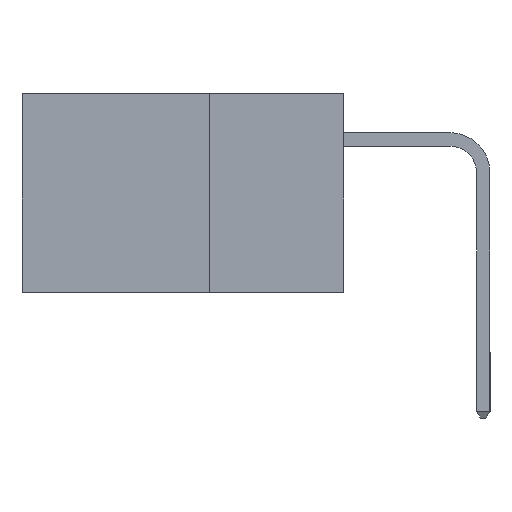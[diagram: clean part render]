
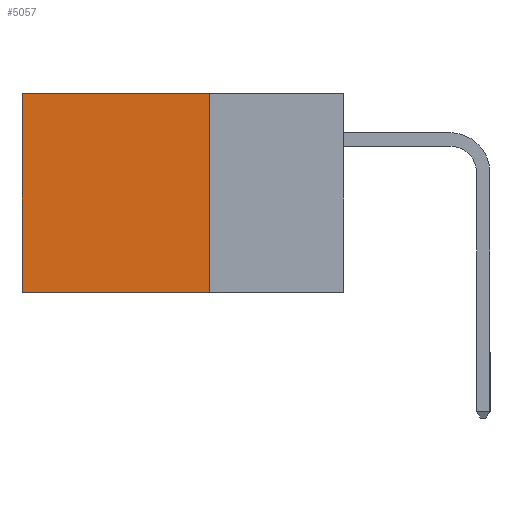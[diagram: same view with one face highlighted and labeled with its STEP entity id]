
A CAD part, left-side view. The second image highlights one B-rep face of the part: STEP entity #5057.
In plain terms, the highlighted planar face has unit normal (-1, 0, 0).
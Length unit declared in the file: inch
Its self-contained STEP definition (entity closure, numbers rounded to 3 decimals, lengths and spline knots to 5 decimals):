
#178 = CARTESIAN_POINT ( 'NONE',  ( 0.2615, 0.6, -0.37 ) ) ;
#509 = CARTESIAN_POINT ( 'NONE',  ( 0.2615, 0.6, 0. ) ) ;
#1676 = DIRECTION ( 'NONE',  ( 0., 0., -1. ) ) ;
#1909 = VERTEX_POINT ( 'NONE', #21114 ) ;
#2066 = LINE ( 'NONE', #12720, #18603 ) ;
#3176 = LINE ( 'NONE', #20677, #4703 ) ;
#3280 = CARTESIAN_POINT ( 'NONE',  ( 0.2615, 0.25, -0.37 ) ) ;
#4654 = DIRECTION ( 'NONE',  ( 0., 1., 0. ) ) ;
#4703 = VECTOR ( 'NONE', #17022, 39.37008 ) ;
#5057 = ADVANCED_FACE ( 'NONE', ( #5669 ), #10710, .F. ) ;
#5129 = EDGE_LOOP ( 'NONE', ( #5294, #18000, #10299, #13114 ) ) ;
#5294 = ORIENTED_EDGE ( 'NONE', *, *, #8417, .T. ) ;
#5669 = FACE_OUTER_BOUND ( 'NONE', #5129, .T. ) ;
#7840 = VECTOR ( 'NONE', #4654, 39.37008 ) ;
#8417 = EDGE_CURVE ( 'NONE', #18795, #21647, #15879, .T. ) ;
#8874 = CARTESIAN_POINT ( 'NONE',  ( 0.2615, 0.25, -0.37 ) ) ;
#9215 = DIRECTION ( 'NONE',  ( 1., 0., 0. ) ) ;
#10299 = ORIENTED_EDGE ( 'NONE', *, *, #20513, .F. ) ;
#10710 = PLANE ( 'NONE',  #16930 ) ;
#10784 = DIRECTION ( 'NONE',  ( 0., 1., 0. ) ) ;
#12720 = CARTESIAN_POINT ( 'NONE',  ( 0.2615, 0.25, 0. ) ) ;
#13114 = ORIENTED_EDGE ( 'NONE', *, *, #20239, .T. ) ;
#13325 = EDGE_CURVE ( 'NONE', #1909, #21647, #17239, .T. ) ;
#13486 = VERTEX_POINT ( 'NONE', #21241 ) ;
#14036 = DIRECTION ( 'NONE',  ( 0., 0., -1. ) ) ;
#15879 = LINE ( 'NONE', #178, #19301 ) ;
#16369 = CARTESIAN_POINT ( 'NONE',  ( 0.2615, 0.6, -0.37 ) ) ;
#16930 = AXIS2_PLACEMENT_3D ( 'NONE', #8874, #9215, #14036 ) ;
#17022 = DIRECTION ( 'NONE',  ( 0., 0., -1. ) ) ;
#17239 = LINE ( 'NONE', #3280, #7840 ) ;
#18000 = ORIENTED_EDGE ( 'NONE', *, *, #13325, .F. ) ;
#18603 = VECTOR ( 'NONE', #10784, 39.37008 ) ;
#18795 = VERTEX_POINT ( 'NONE', #509 ) ;
#19301 = VECTOR ( 'NONE', #1676, 39.37008 ) ;
#20239 = EDGE_CURVE ( 'NONE', #13486, #18795, #2066, .T. ) ;
#20513 = EDGE_CURVE ( 'NONE', #13486, #1909, #3176, .T. ) ;
#20677 = CARTESIAN_POINT ( 'NONE',  ( 0.2615, 0.25, -0.37 ) ) ;
#21114 = CARTESIAN_POINT ( 'NONE',  ( 0.2615, 0.25, -0.37 ) ) ;
#21241 = CARTESIAN_POINT ( 'NONE',  ( 0.2615, 0.25, 0. ) ) ;
#21647 = VERTEX_POINT ( 'NONE', #16369 ) ;
